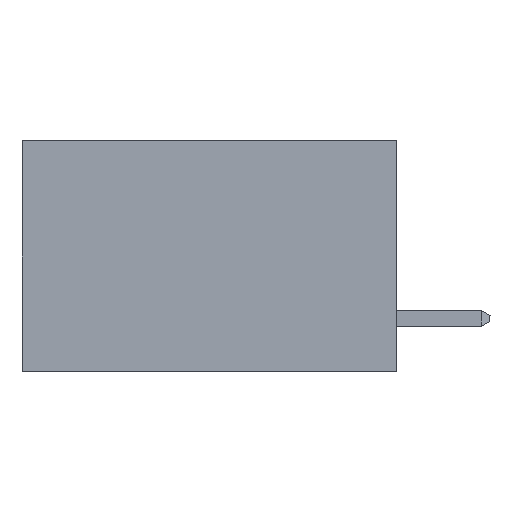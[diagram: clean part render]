
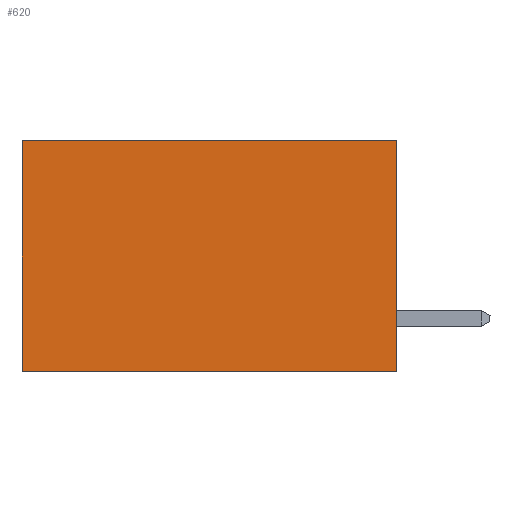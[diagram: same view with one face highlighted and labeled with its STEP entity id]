
A CAD part, left-side view. The second image highlights one B-rep face of the part: STEP entity #620.
In plain terms, the highlighted planar face has unit normal (-1, 0, 0).
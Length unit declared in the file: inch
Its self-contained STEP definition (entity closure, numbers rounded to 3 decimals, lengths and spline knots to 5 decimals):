
#400 = VECTOR ( 'NONE', #4807, 39.37008 ) ;
#620 = ADVANCED_FACE ( 'NONE', ( #19080 ), #18611, .F. ) ;
#942 = CARTESIAN_POINT ( 'NONE',  ( 0.2615, 0., -0.37 ) ) ;
#1311 = LINE ( 'NONE', #14520, #16573 ) ;
#1393 = ORIENTED_EDGE ( 'NONE', *, *, #5464, .T. ) ;
#1698 = DIRECTION ( 'NONE',  ( 0., 1., 0. ) ) ;
#2069 = LINE ( 'NONE', #15275, #15747 ) ;
#2409 = EDGE_CURVE ( 'NONE', #9365, #10584, #1311, .T. ) ;
#4684 = LINE ( 'NONE', #10402, #11489 ) ;
#4807 = DIRECTION ( 'NONE',  ( 0., 0., -1. ) ) ;
#5464 = EDGE_CURVE ( 'NONE', #9365, #7159, #2069, .T. ) ;
#6995 = ORIENTED_EDGE ( 'NONE', *, *, #2409, .F. ) ;
#7159 = VERTEX_POINT ( 'NONE', #12079 ) ;
#7707 = CARTESIAN_POINT ( 'NONE',  ( 0.2615, 0.6, -0.37 ) ) ;
#8010 = CARTESIAN_POINT ( 'NONE',  ( 0.2615, 0.6, -0.37 ) ) ;
#8594 = DIRECTION ( 'NONE',  ( 0., 0., -1. ) ) ;
#8608 = VERTEX_POINT ( 'NONE', #8010 ) ;
#9365 = VERTEX_POINT ( 'NONE', #14612 ) ;
#10402 = CARTESIAN_POINT ( 'NONE',  ( 0.2615, 0., -0.37 ) ) ;
#10584 = VERTEX_POINT ( 'NONE', #942 ) ;
#11450 = EDGE_LOOP ( 'NONE', ( #16048, #14712, #6995, #1393 ) ) ;
#11489 = VECTOR ( 'NONE', #14860, 39.37008 ) ;
#12079 = CARTESIAN_POINT ( 'NONE',  ( 0.2615, 0.6, 0. ) ) ;
#14520 = CARTESIAN_POINT ( 'NONE',  ( 0.2615, 0., -0.37 ) ) ;
#14531 = AXIS2_PLACEMENT_3D ( 'NONE', #14724, #18707, #15717 ) ;
#14612 = CARTESIAN_POINT ( 'NONE',  ( 0.2615, 0., 0. ) ) ;
#14712 = ORIENTED_EDGE ( 'NONE', *, *, #14926, .F. ) ;
#14724 = CARTESIAN_POINT ( 'NONE',  ( 0.2615, 0., -0.37 ) ) ;
#14860 = DIRECTION ( 'NONE',  ( 0., 1., 0. ) ) ;
#14926 = EDGE_CURVE ( 'NONE', #10584, #8608, #4684, .T. ) ;
#15275 = CARTESIAN_POINT ( 'NONE',  ( 0.2615, 0., 0. ) ) ;
#15717 = DIRECTION ( 'NONE',  ( 0., 0., -1. ) ) ;
#15747 = VECTOR ( 'NONE', #1698, 39.37008 ) ;
#16048 = ORIENTED_EDGE ( 'NONE', *, *, #17803, .T. ) ;
#16573 = VECTOR ( 'NONE', #8594, 39.37008 ) ;
#17803 = EDGE_CURVE ( 'NONE', #7159, #8608, #18347, .T. ) ;
#18347 = LINE ( 'NONE', #7707, #400 ) ;
#18611 = PLANE ( 'NONE',  #14531 ) ;
#18707 = DIRECTION ( 'NONE',  ( 1., 0., 0. ) ) ;
#19080 = FACE_OUTER_BOUND ( 'NONE', #11450, .T. ) ;
